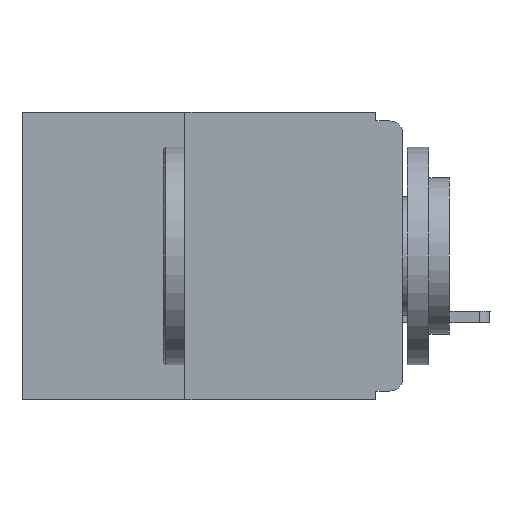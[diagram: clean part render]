
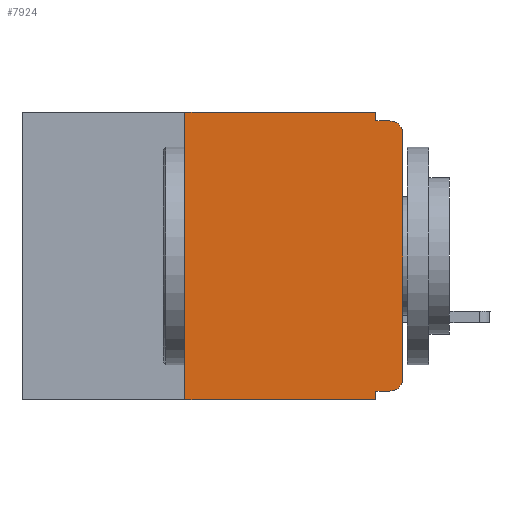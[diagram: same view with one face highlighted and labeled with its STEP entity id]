
A CAD part, left-side view. The second image highlights one B-rep face of the part: STEP entity #7924.
In plain terms, the highlighted planar face has unit normal (-1, 0, 0).
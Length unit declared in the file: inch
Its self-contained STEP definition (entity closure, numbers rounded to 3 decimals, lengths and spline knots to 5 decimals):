
#9 = CARTESIAN_POINT ( 'NONE',  ( 0., 0.031, -0.32 ) ) ;
#195 = ORIENTED_EDGE ( 'NONE', *, *, #6786, .T. ) ;
#304 = VERTEX_POINT ( 'NONE', #2767 ) ;
#744 = ORIENTED_EDGE ( 'NONE', *, *, #10609, .T. ) ;
#870 = DIRECTION ( 'NONE',  ( 0., 1., 0. ) ) ;
#1128 = CARTESIAN_POINT ( 'NONE',  ( 0., 0.25, -0.33 ) ) ;
#1175 = CARTESIAN_POINT ( 'NONE',  ( 0., 0.031, 0. ) ) ;
#1210 = DIRECTION ( 'NONE',  ( 0., 0., -1. ) ) ;
#1310 = CARTESIAN_POINT ( 'NONE',  ( 0., 0.015, -0.01 ) ) ;
#1314 = LINE ( 'NONE', #10171, #10134 ) ;
#1509 = CARTESIAN_POINT ( 'NONE',  ( 0., 0.25, -0.33 ) ) ;
#1511 = DIRECTION ( 'NONE',  ( 0., 0., -1. ) ) ;
#1519 = VERTEX_POINT ( 'NONE', #2335 ) ;
#1536 = VERTEX_POINT ( 'NONE', #4201 ) ;
#1691 = LINE ( 'NONE', #3577, #6298 ) ;
#1803 = VECTOR ( 'NONE', #9075, 39.37008 ) ;
#1846 = DIRECTION ( 'NONE',  ( 0., -1., 0. ) ) ;
#1894 = CIRCLE ( 'NONE', #4861, 0.015 ) ;
#1916 = CARTESIAN_POINT ( 'NONE',  ( 0., 0.015, -0.32 ) ) ;
#2178 = ORIENTED_EDGE ( 'NONE', *, *, #3599, .F. ) ;
#2335 = CARTESIAN_POINT ( 'NONE',  ( 0., 0.25, 0. ) ) ;
#2349 = DIRECTION ( 'NONE',  ( 1., 0., 0. ) ) ;
#2390 = DIRECTION ( 'NONE',  ( 0., 0., -1. ) ) ;
#2427 = CARTESIAN_POINT ( 'NONE',  ( 0., 0., -0.025 ) ) ;
#2432 = FACE_OUTER_BOUND ( 'NONE', #6095, .T. ) ;
#2661 = CARTESIAN_POINT ( 'NONE',  ( 0., 0., -0.32 ) ) ;
#2683 = EDGE_CURVE ( 'NONE', #8739, #1536, #10360, .T. ) ;
#2767 = CARTESIAN_POINT ( 'NONE',  ( 0., 0., -0.305 ) ) ;
#2785 = LINE ( 'NONE', #9037, #1803 ) ;
#2870 = VERTEX_POINT ( 'NONE', #1916 ) ;
#3054 = DIRECTION ( 'NONE',  ( -1., 0., 0. ) ) ;
#3132 = CARTESIAN_POINT ( 'NONE',  ( 0., 0.015, -0.025 ) ) ;
#3339 = CARTESIAN_POINT ( 'NONE',  ( 0., 0.031, 0. ) ) ;
#3577 = CARTESIAN_POINT ( 'NONE',  ( 0., 0., 0. ) ) ;
#3599 = EDGE_CURVE ( 'NONE', #5803, #1519, #6016, .T. ) ;
#3635 = ORIENTED_EDGE ( 'NONE', *, *, #4624, .T. ) ;
#3876 = ORIENTED_EDGE ( 'NONE', *, *, #8634, .F. ) ;
#4106 = VERTEX_POINT ( 'NONE', #9467 ) ;
#4200 = CARTESIAN_POINT ( 'NONE',  ( 0., 0.437, 0. ) ) ;
#4201 = CARTESIAN_POINT ( 'NONE',  ( 0., 0.031, -0.33 ) ) ;
#4214 = VECTOR ( 'NONE', #870, 39.37008 ) ;
#4304 = ORIENTED_EDGE ( 'NONE', *, *, #7119, .T. ) ;
#4364 = EDGE_CURVE ( 'NONE', #4106, #10345, #2785, .T. ) ;
#4439 = LINE ( 'NONE', #4200, #10809 ) ;
#4483 = ORIENTED_EDGE ( 'NONE', *, *, #4978, .F. ) ;
#4531 = AXIS2_PLACEMENT_3D ( 'NONE', #11659, #2349, #2390 ) ;
#4592 = LINE ( 'NONE', #3339, #8382 ) ;
#4624 = EDGE_CURVE ( 'NONE', #2870, #304, #6702, .T. ) ;
#4861 = AXIS2_PLACEMENT_3D ( 'NONE', #3132, #3054, #11355 ) ;
#4978 = EDGE_CURVE ( 'NONE', #2870, #8739, #6111, .T. ) ;
#5089 = ORIENTED_EDGE ( 'NONE', *, *, #4364, .F. ) ;
#5122 = DIRECTION ( 'NONE',  ( 0., -1., 0. ) ) ;
#5803 = VERTEX_POINT ( 'NONE', #1509 ) ;
#6016 = LINE ( 'NONE', #1128, #10628 ) ;
#6092 = PLANE ( 'NONE',  #4531 ) ;
#6095 = EDGE_LOOP ( 'NONE', ( #744, #4304, #5089, #3876, #8101, #2178, #195, #8990, #4483, #3635 ) ) ;
#6111 = LINE ( 'NONE', #2661, #4214 ) ;
#6298 = VECTOR ( 'NONE', #9065, 39.37008 ) ;
#6702 = CIRCLE ( 'NONE', #7578, 0.015 ) ;
#6786 = EDGE_CURVE ( 'NONE', #5803, #1536, #1314, .T. ) ;
#6903 = VECTOR ( 'NONE', #7373, 39.37008 ) ;
#7104 = VERTEX_POINT ( 'NONE', #1175 ) ;
#7119 = EDGE_CURVE ( 'NONE', #9705, #10345, #1894, .T. ) ;
#7373 = DIRECTION ( 'NONE',  ( 0., 0., -1. ) ) ;
#7578 = AXIS2_PLACEMENT_3D ( 'NONE', #11427, #8609, #1210 ) ;
#7729 = DIRECTION ( 'NONE',  ( 0., 0., 1. ) ) ;
#7924 = ADVANCED_FACE ( 'NONE', ( #2432 ), #6092, .F. ) ;
#8101 = ORIENTED_EDGE ( 'NONE', *, *, #8651, .F. ) ;
#8382 = VECTOR ( 'NONE', #1511, 39.37008 ) ;
#8609 = DIRECTION ( 'NONE',  ( -1., 0., 0. ) ) ;
#8634 = EDGE_CURVE ( 'NONE', #7104, #4106, #4592, .T. ) ;
#8651 = EDGE_CURVE ( 'NONE', #1519, #7104, #4439, .T. ) ;
#8739 = VERTEX_POINT ( 'NONE', #9 ) ;
#8990 = ORIENTED_EDGE ( 'NONE', *, *, #2683, .F. ) ;
#9037 = CARTESIAN_POINT ( 'NONE',  ( 0., 0., -0.01 ) ) ;
#9065 = DIRECTION ( 'NONE',  ( 0., 0., 1. ) ) ;
#9075 = DIRECTION ( 'NONE',  ( 0., -1., 0. ) ) ;
#9467 = CARTESIAN_POINT ( 'NONE',  ( 0., 0.031, -0.01 ) ) ;
#9705 = VERTEX_POINT ( 'NONE', #2427 ) ;
#10134 = VECTOR ( 'NONE', #1846, 39.37008 ) ;
#10171 = CARTESIAN_POINT ( 'NONE',  ( 0., 0.437, -0.33 ) ) ;
#10345 = VERTEX_POINT ( 'NONE', #1310 ) ;
#10360 = LINE ( 'NONE', #10989, #6903 ) ;
#10609 = EDGE_CURVE ( 'NONE', #304, #9705, #1691, .T. ) ;
#10628 = VECTOR ( 'NONE', #7729, 39.37008 ) ;
#10809 = VECTOR ( 'NONE', #5122, 39.37008 ) ;
#10989 = CARTESIAN_POINT ( 'NONE',  ( 0., 0.031, -0.33 ) ) ;
#11355 = DIRECTION ( 'NONE',  ( 0., 0., -1. ) ) ;
#11427 = CARTESIAN_POINT ( 'NONE',  ( 0., 0.015, -0.305 ) ) ;
#11659 = CARTESIAN_POINT ( 'NONE',  ( 0., 0.437, 0. ) ) ;
